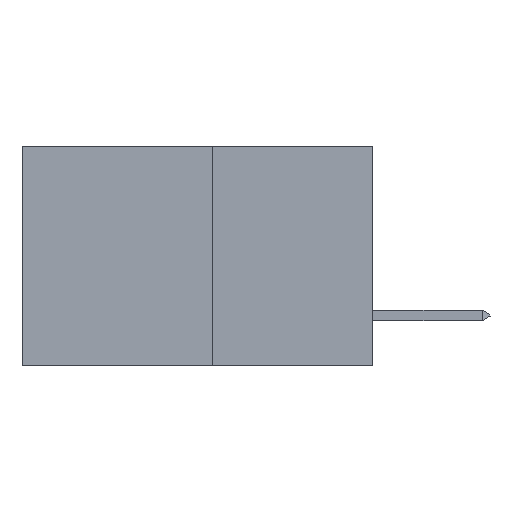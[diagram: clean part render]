
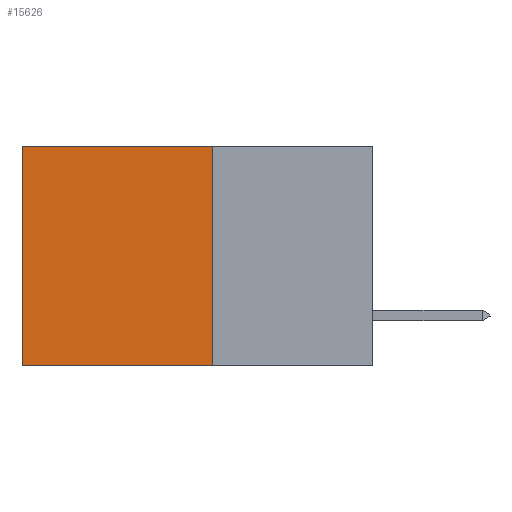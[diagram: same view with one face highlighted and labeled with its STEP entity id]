
A CAD part, left-side view. The second image highlights one B-rep face of the part: STEP entity #15626.
In plain terms, the highlighted planar face has unit normal (-1, 0, 0).
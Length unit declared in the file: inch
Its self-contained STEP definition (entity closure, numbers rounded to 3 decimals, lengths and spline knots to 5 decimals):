
#1015 = ORIENTED_EDGE ( 'NONE', *, *, #24201, .T. ) ;
#1819 = AXIS2_PLACEMENT_3D ( 'NONE', #20801, #16953, #4934 ) ;
#2115 = CARTESIAN_POINT ( 'NONE',  ( 0.277, 0.59, -0.37 ) ) ;
#2709 = ORIENTED_EDGE ( 'NONE', *, *, #24315, .F. ) ;
#4024 = FACE_OUTER_BOUND ( 'NONE', #19240, .T. ) ;
#4531 = VECTOR ( 'NONE', #8689, 39.37008 ) ;
#4934 = DIRECTION ( 'NONE',  ( 0., 0., -1. ) ) ;
#5929 = VERTEX_POINT ( 'NONE', #2115 ) ;
#6799 = LINE ( 'NONE', #20107, #12164 ) ;
#6802 = EDGE_CURVE ( 'NONE', #17381, #17741, #15227, .T. ) ;
#6872 = CARTESIAN_POINT ( 'NONE',  ( 0.277, 0.27, -0.37 ) ) ;
#8595 = DIRECTION ( 'NONE',  ( 0., 1., 0. ) ) ;
#8689 = DIRECTION ( 'NONE',  ( 0., 1., 0. ) ) ;
#9923 = CARTESIAN_POINT ( 'NONE',  ( 0.277, 0.27, 0. ) ) ;
#10254 = LINE ( 'NONE', #14507, #20176 ) ;
#10557 = DIRECTION ( 'NONE',  ( 0., 0., -1. ) ) ;
#12164 = VECTOR ( 'NONE', #22076, 39.37008 ) ;
#12814 = EDGE_CURVE ( 'NONE', #20559, #5929, #19480, .T. ) ;
#12960 = PLANE ( 'NONE',  #1819 ) ;
#14507 = CARTESIAN_POINT ( 'NONE',  ( 0.277, 0.27, -0.37 ) ) ;
#15227 = LINE ( 'NONE', #9923, #4531 ) ;
#15547 = CARTESIAN_POINT ( 'NONE',  ( 0.277, 0.59, 0. ) ) ;
#15626 = ADVANCED_FACE ( 'NONE', ( #4024 ), #12960, .F. ) ;
#16538 = CARTESIAN_POINT ( 'NONE',  ( 0.277, 0.27, -0.37 ) ) ;
#16953 = DIRECTION ( 'NONE',  ( 1., 0., 0. ) ) ;
#17381 = VERTEX_POINT ( 'NONE', #18497 ) ;
#17741 = VERTEX_POINT ( 'NONE', #15547 ) ;
#18497 = CARTESIAN_POINT ( 'NONE',  ( 0.277, 0.27, 0. ) ) ;
#19240 = EDGE_LOOP ( 'NONE', ( #1015, #23557, #2709, #23360 ) ) ;
#19480 = LINE ( 'NONE', #16538, #24648 ) ;
#20107 = CARTESIAN_POINT ( 'NONE',  ( 0.277, 0.59, -0.37 ) ) ;
#20176 = VECTOR ( 'NONE', #10557, 39.37008 ) ;
#20559 = VERTEX_POINT ( 'NONE', #6872 ) ;
#20801 = CARTESIAN_POINT ( 'NONE',  ( 0.277, 0.27, -0.37 ) ) ;
#22076 = DIRECTION ( 'NONE',  ( 0., 0., -1. ) ) ;
#23360 = ORIENTED_EDGE ( 'NONE', *, *, #6802, .T. ) ;
#23557 = ORIENTED_EDGE ( 'NONE', *, *, #12814, .F. ) ;
#24201 = EDGE_CURVE ( 'NONE', #17741, #5929, #6799, .T. ) ;
#24315 = EDGE_CURVE ( 'NONE', #17381, #20559, #10254, .T. ) ;
#24648 = VECTOR ( 'NONE', #8595, 39.37008 ) ;
